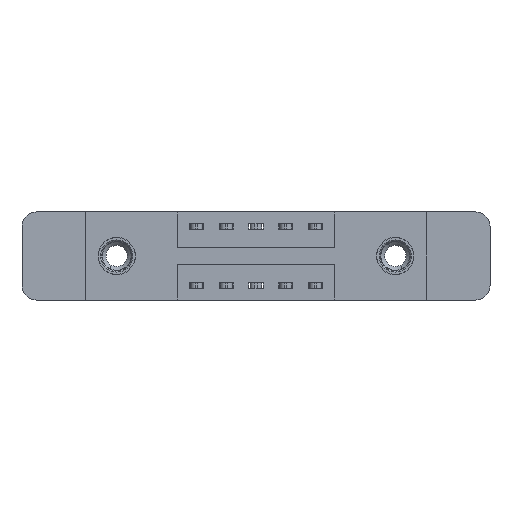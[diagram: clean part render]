
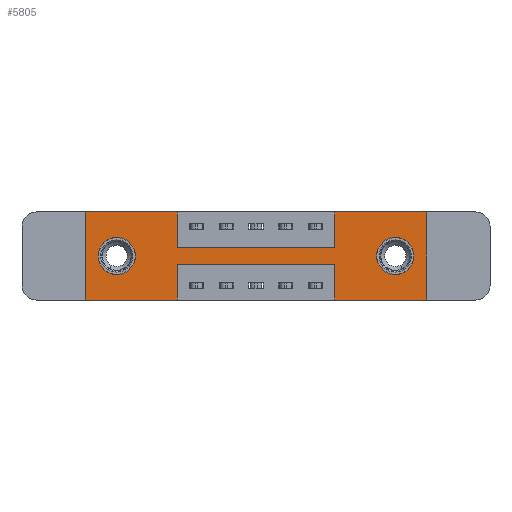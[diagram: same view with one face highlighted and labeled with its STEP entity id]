
A CAD part, front view. The second image highlights one B-rep face of the part: STEP entity #5805.
In plain terms, the highlighted planar face has unit normal (0, -1, 0).
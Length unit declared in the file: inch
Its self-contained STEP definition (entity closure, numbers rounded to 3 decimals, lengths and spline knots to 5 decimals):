
#214 = VECTOR ( 'NONE', #12599, 39.37008 ) ;
#268 = CIRCLE ( 'NONE', #10093, 0.078 ) ;
#271 = ORIENTED_EDGE ( 'NONE', *, *, #12580, .F. ) ;
#275 = EDGE_CURVE ( 'NONE', #376, #10108, #7095, .T. ) ;
#376 = VERTEX_POINT ( 'NONE', #12529 ) ;
#554 = DIRECTION ( 'NONE',  ( 0., 0., -1. ) ) ;
#577 = DIRECTION ( 'NONE',  ( 0., 0., -1. ) ) ;
#601 = DIRECTION ( 'NONE',  ( 0., 0., -1. ) ) ;
#847 = CARTESIAN_POINT ( 'NONE',  ( 0.1325, 0., -0.185 ) ) ;
#911 = CARTESIAN_POINT ( 'NONE',  ( 1.435, 0., 0. ) ) ;
#926 = CARTESIAN_POINT ( 'NONE',  ( 1.0475, 0., 0. ) ) ;
#983 = ORIENTED_EDGE ( 'NONE', *, *, #8778, .F. ) ;
#1167 = ORIENTED_EDGE ( 'NONE', *, *, #3475, .T. ) ;
#1336 = VERTEX_POINT ( 'NONE', #12586 ) ;
#1666 = CARTESIAN_POINT ( 'NONE',  ( 0.3875, 0., 0. ) ) ;
#1805 = CARTESIAN_POINT ( 'NONE',  ( 1.3025, 0., -0.185 ) ) ;
#1834 = CARTESIAN_POINT ( 'NONE',  ( 1.3025, 0., -0.107 ) ) ;
#1883 = CARTESIAN_POINT ( 'NONE',  ( 1.0475, 0., -0.37 ) ) ;
#2058 = ORIENTED_EDGE ( 'NONE', *, *, #5258, .F. ) ;
#2311 = VERTEX_POINT ( 'NONE', #7652 ) ;
#2379 = LINE ( 'NONE', #6625, #2669 ) ;
#2457 = VECTOR ( 'NONE', #8755, 39.37008 ) ;
#2531 = EDGE_CURVE ( 'NONE', #9400, #6241, #10031, .T. ) ;
#2581 = CARTESIAN_POINT ( 'NONE',  ( 0.3875, 0., -0.15 ) ) ;
#2590 = VERTEX_POINT ( 'NONE', #4874 ) ;
#2630 = CARTESIAN_POINT ( 'NONE',  ( 0., 0., -0.37 ) ) ;
#2669 = VECTOR ( 'NONE', #10895, 39.37008 ) ;
#2688 = LINE ( 'NONE', #1666, #10272 ) ;
#2710 = LINE ( 'NONE', #2630, #8315 ) ;
#2735 = ORIENTED_EDGE ( 'NONE', *, *, #275, .F. ) ;
#2802 = CARTESIAN_POINT ( 'NONE',  ( 0., 0., 0. ) ) ;
#2895 = ORIENTED_EDGE ( 'NONE', *, *, #11772, .T. ) ;
#2991 = ORIENTED_EDGE ( 'NONE', *, *, #4772, .F. ) ;
#3086 = ORIENTED_EDGE ( 'NONE', *, *, #5727, .F. ) ;
#3145 = CARTESIAN_POINT ( 'NONE',  ( 0.1325, 0., -0.263 ) ) ;
#3233 = DIRECTION ( 'NONE',  ( 0., 1., 0. ) ) ;
#3319 = ORIENTED_EDGE ( 'NONE', *, *, #6641, .F. ) ;
#3400 = EDGE_CURVE ( 'NONE', #12207, #4837, #268, .T. ) ;
#3475 = EDGE_CURVE ( 'NONE', #6241, #9400, #6958, .T. ) ;
#3544 = DIRECTION ( 'NONE',  ( 0., 0., -1. ) ) ;
#3566 = VECTOR ( 'NONE', #5131, 39.37008 ) ;
#3849 = AXIS2_PLACEMENT_3D ( 'NONE', #9012, #9924, #554 ) ;
#4030 = VERTEX_POINT ( 'NONE', #4672 ) ;
#4069 = VERTEX_POINT ( 'NONE', #2581 ) ;
#4072 = AXIS2_PLACEMENT_3D ( 'NONE', #10911, #3233, #5579 ) ;
#4577 = DIRECTION ( 'NONE',  ( 0., 0., 1. ) ) ;
#4672 = CARTESIAN_POINT ( 'NONE',  ( 1.0475, 0., -0.37 ) ) ;
#4771 = DIRECTION ( 'NONE',  ( 0., 0., 1. ) ) ;
#4772 = EDGE_CURVE ( 'NONE', #7236, #13578, #12080, .T. ) ;
#4837 = VERTEX_POINT ( 'NONE', #8973 ) ;
#4874 = CARTESIAN_POINT ( 'NONE',  ( 0.3875, 0., -0.22 ) ) ;
#4889 = CARTESIAN_POINT ( 'NONE',  ( 1.3025, 0., -0.185 ) ) ;
#4942 = ORIENTED_EDGE ( 'NONE', *, *, #12014, .F. ) ;
#5131 = DIRECTION ( 'NONE',  ( 0., 0., -1. ) ) ;
#5258 = EDGE_CURVE ( 'NONE', #12613, #7236, #9030, .T. ) ;
#5563 = EDGE_LOOP ( 'NONE', ( #10537, #2895 ) ) ;
#5579 = DIRECTION ( 'NONE',  ( 0., 0., 1. ) ) ;
#5727 = EDGE_CURVE ( 'NONE', #10108, #4030, #2710, .T. ) ;
#5805 = ADVANCED_FACE ( 'NONE', ( #8850, #11017, #5822 ), #10131, .T. ) ;
#5822 = FACE_OUTER_BOUND ( 'NONE', #9766, .T. ) ;
#5842 = CARTESIAN_POINT ( 'NONE',  ( 0., 0., -0.37 ) ) ;
#5932 = CARTESIAN_POINT ( 'NONE',  ( 0., 0., 0. ) ) ;
#6241 = VERTEX_POINT ( 'NONE', #10092 ) ;
#6430 = AXIS2_PLACEMENT_3D ( 'NONE', #4889, #7050, #577 ) ;
#6462 = VECTOR ( 'NONE', #7234, 39.37008 ) ;
#6513 = CARTESIAN_POINT ( 'NONE',  ( 0.3875, 0., -0.22 ) ) ;
#6625 = CARTESIAN_POINT ( 'NONE',  ( 0., 0., 0. ) ) ;
#6634 = LINE ( 'NONE', #6513, #2457 ) ;
#6641 = EDGE_CURVE ( 'NONE', #9646, #376, #2379, .T. ) ;
#6958 = CIRCLE ( 'NONE', #4072, 0.078 ) ;
#7019 = ORIENTED_EDGE ( 'NONE', *, *, #9005, .F. ) ;
#7050 = DIRECTION ( 'NONE',  ( 0., 1., 0. ) ) ;
#7058 = DIRECTION ( 'NONE',  ( 1., 0., 0. ) ) ;
#7095 = LINE ( 'NONE', #911, #3566 ) ;
#7221 = VECTOR ( 'NONE', #10207, 39.37008 ) ;
#7234 = DIRECTION ( 'NONE',  ( 1., 0., 0. ) ) ;
#7236 = VERTEX_POINT ( 'NONE', #12265 ) ;
#7239 = LINE ( 'NONE', #1883, #214 ) ;
#7257 = DIRECTION ( 'NONE',  ( 0., 1., 0. ) ) ;
#7435 = EDGE_CURVE ( 'NONE', #4030, #1336, #7239, .T. ) ;
#7652 = CARTESIAN_POINT ( 'NONE',  ( 1.0475, 0., -0.15 ) ) ;
#8025 = DIRECTION ( 'NONE',  ( -1., 0., 0. ) ) ;
#8107 = CARTESIAN_POINT ( 'NONE',  ( 0.3875, 0., -0.37 ) ) ;
#8315 = VECTOR ( 'NONE', #8025, 39.37008 ) ;
#8567 = CARTESIAN_POINT ( 'NONE',  ( 1.435, 0., -0.37 ) ) ;
#8755 = DIRECTION ( 'NONE',  ( -1., 0., 0. ) ) ;
#8778 = EDGE_CURVE ( 'NONE', #13779, #4069, #2688, .T. ) ;
#8841 = ORIENTED_EDGE ( 'NONE', *, *, #12512, .F. ) ;
#8850 = FACE_BOUND ( 'NONE', #5563, .T. ) ;
#8940 = LINE ( 'NONE', #8107, #10881 ) ;
#8973 = CARTESIAN_POINT ( 'NONE',  ( 1.3025, 0., -0.263 ) ) ;
#9005 = EDGE_CURVE ( 'NONE', #1336, #2590, #6634, .T. ) ;
#9012 = CARTESIAN_POINT ( 'NONE',  ( 0., 0., -0.37 ) ) ;
#9030 = LINE ( 'NONE', #5842, #7221 ) ;
#9295 = EDGE_CURVE ( 'NONE', #13578, #13779, #12367, .T. ) ;
#9296 = DIRECTION ( 'NONE',  ( 0., 0., 1. ) ) ;
#9400 = VERTEX_POINT ( 'NONE', #3145 ) ;
#9646 = VERTEX_POINT ( 'NONE', #926 ) ;
#9756 = CARTESIAN_POINT ( 'NONE',  ( 0.3875, 0., 0. ) ) ;
#9766 = EDGE_LOOP ( 'NONE', ( #4942, #7019, #9880, #3086, #2735, #3319, #8841, #271, #983, #10134, #2991, #2058 ) ) ;
#9880 = ORIENTED_EDGE ( 'NONE', *, *, #7435, .F. ) ;
#9924 = DIRECTION ( 'NONE',  ( 0., -1., 0. ) ) ;
#10031 = CIRCLE ( 'NONE', #12005, 0.078 ) ;
#10032 = ORIENTED_EDGE ( 'NONE', *, *, #2531, .T. ) ;
#10047 = CARTESIAN_POINT ( 'NONE',  ( 1.0475, 0., 0. ) ) ;
#10092 = CARTESIAN_POINT ( 'NONE',  ( 0.1325, 0., -0.107 ) ) ;
#10093 = AXIS2_PLACEMENT_3D ( 'NONE', #1805, #10380, #10585 ) ;
#10108 = VERTEX_POINT ( 'NONE', #8567 ) ;
#10131 = PLANE ( 'NONE',  #3849 ) ;
#10134 = ORIENTED_EDGE ( 'NONE', *, *, #9295, .F. ) ;
#10207 = DIRECTION ( 'NONE',  ( -1., 0., 0. ) ) ;
#10272 = VECTOR ( 'NONE', #601, 39.37008 ) ;
#10380 = DIRECTION ( 'NONE',  ( 0., 1., 0. ) ) ;
#10388 = CARTESIAN_POINT ( 'NONE',  ( 0.3875, 0., -0.37 ) ) ;
#10537 = ORIENTED_EDGE ( 'NONE', *, *, #3400, .T. ) ;
#10585 = DIRECTION ( 'NONE',  ( 0., 0., -1. ) ) ;
#10881 = VECTOR ( 'NONE', #3544, 39.37008 ) ;
#10895 = DIRECTION ( 'NONE',  ( 1., 0., 0. ) ) ;
#10911 = CARTESIAN_POINT ( 'NONE',  ( 0.1325, 0., -0.185 ) ) ;
#11011 = CARTESIAN_POINT ( 'NONE',  ( 0., 0., 0. ) ) ;
#11017 = FACE_BOUND ( 'NONE', #13199, .T. ) ;
#11555 = LINE ( 'NONE', #12456, #6462 ) ;
#11772 = EDGE_CURVE ( 'NONE', #4837, #12207, #12450, .T. ) ;
#11967 = LINE ( 'NONE', #10047, #11972 ) ;
#11972 = VECTOR ( 'NONE', #4577, 39.37008 ) ;
#12005 = AXIS2_PLACEMENT_3D ( 'NONE', #847, #7257, #9296 ) ;
#12014 = EDGE_CURVE ( 'NONE', #2590, #12613, #8940, .T. ) ;
#12080 = LINE ( 'NONE', #5932, #12099 ) ;
#12099 = VECTOR ( 'NONE', #4771, 39.37008 ) ;
#12207 = VERTEX_POINT ( 'NONE', #1834 ) ;
#12221 = VECTOR ( 'NONE', #7058, 39.37008 ) ;
#12265 = CARTESIAN_POINT ( 'NONE',  ( 0., 0., -0.37 ) ) ;
#12367 = LINE ( 'NONE', #2802, #12221 ) ;
#12450 = CIRCLE ( 'NONE', #6430, 0.078 ) ;
#12456 = CARTESIAN_POINT ( 'NONE',  ( 0.3875, 0., -0.15 ) ) ;
#12512 = EDGE_CURVE ( 'NONE', #2311, #9646, #11967, .T. ) ;
#12529 = CARTESIAN_POINT ( 'NONE',  ( 1.435, 0., 0. ) ) ;
#12580 = EDGE_CURVE ( 'NONE', #4069, #2311, #11555, .T. ) ;
#12586 = CARTESIAN_POINT ( 'NONE',  ( 1.0475, 0., -0.22 ) ) ;
#12599 = DIRECTION ( 'NONE',  ( 0., 0., 1. ) ) ;
#12613 = VERTEX_POINT ( 'NONE', #10388 ) ;
#13199 = EDGE_LOOP ( 'NONE', ( #1167, #10032 ) ) ;
#13578 = VERTEX_POINT ( 'NONE', #11011 ) ;
#13779 = VERTEX_POINT ( 'NONE', #9756 ) ;
